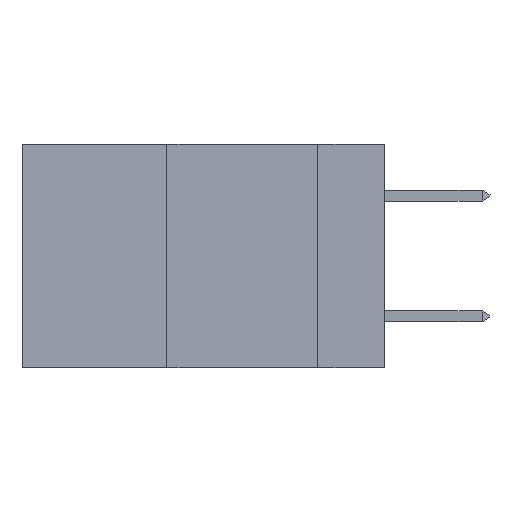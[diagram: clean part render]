
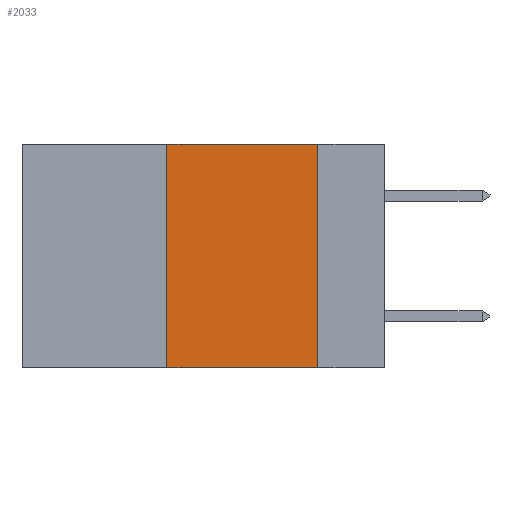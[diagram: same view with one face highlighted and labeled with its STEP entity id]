
A CAD part, left-side view. The second image highlights one B-rep face of the part: STEP entity #2033.
In plain terms, the highlighted planar face has unit normal (-1, 0, 0).
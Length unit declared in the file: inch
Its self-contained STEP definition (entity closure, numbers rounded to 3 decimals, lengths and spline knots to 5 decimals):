
#476 = VECTOR ( 'NONE', #6105, 39.37008 ) ;
#523 = CARTESIAN_POINT ( 'NONE',  ( 0., 0.11, 0. ) ) ;
#810 = ORIENTED_EDGE ( 'NONE', *, *, #3979, .F. ) ;
#1506 = DIRECTION ( 'NONE',  ( 0., 0., -1. ) ) ;
#2033 = ADVANCED_FACE ( 'NONE', ( #2945 ), #10459, .F. ) ;
#2602 = CARTESIAN_POINT ( 'NONE',  ( 0., 0.11, 0. ) ) ;
#2945 = FACE_OUTER_BOUND ( 'NONE', #3031, .T. ) ;
#3031 = EDGE_LOOP ( 'NONE', ( #9887, #810, #5860, #4939 ) ) ;
#3814 = DIRECTION ( 'NONE',  ( 0., -1., 0. ) ) ;
#3979 = EDGE_CURVE ( 'NONE', #7374, #7402, #9338, .T. ) ;
#4024 = VECTOR ( 'NONE', #5511, 39.37008 ) ;
#4125 = VECTOR ( 'NONE', #8876, 39.37008 ) ;
#4846 = EDGE_CURVE ( 'NONE', #8097, #7374, #6092, .T. ) ;
#4939 = ORIENTED_EDGE ( 'NONE', *, *, #6793, .T. ) ;
#5511 = DIRECTION ( 'NONE',  ( 0., 0., 1. ) ) ;
#5563 = CARTESIAN_POINT ( 'NONE',  ( 0., 0.6, 0. ) ) ;
#5622 = VERTEX_POINT ( 'NONE', #10888 ) ;
#5860 = ORIENTED_EDGE ( 'NONE', *, *, #4846, .F. ) ;
#6067 = CARTESIAN_POINT ( 'NONE',  ( 0., 0.36, -0.37 ) ) ;
#6092 = LINE ( 'NONE', #10984, #4024 ) ;
#6105 = DIRECTION ( 'NONE',  ( 0., 0., -1. ) ) ;
#6523 = CARTESIAN_POINT ( 'NONE',  ( 0., 0.6, -0.37 ) ) ;
#6793 = EDGE_CURVE ( 'NONE', #8097, #5622, #10842, .T. ) ;
#7257 = VECTOR ( 'NONE', #3814, 39.37008 ) ;
#7374 = VERTEX_POINT ( 'NONE', #7757 ) ;
#7402 = VERTEX_POINT ( 'NONE', #2602 ) ;
#7448 = LINE ( 'NONE', #523, #476 ) ;
#7757 = CARTESIAN_POINT ( 'NONE',  ( 0., 0.36, 0. ) ) ;
#8097 = VERTEX_POINT ( 'NONE', #6067 ) ;
#8160 = EDGE_CURVE ( 'NONE', #7402, #5622, #7448, .T. ) ;
#8876 = DIRECTION ( 'NONE',  ( 0., -1., 0. ) ) ;
#9103 = AXIS2_PLACEMENT_3D ( 'NONE', #10654, #10418, #1506 ) ;
#9338 = LINE ( 'NONE', #5563, #7257 ) ;
#9887 = ORIENTED_EDGE ( 'NONE', *, *, #8160, .F. ) ;
#10418 = DIRECTION ( 'NONE',  ( 1., 0., 0. ) ) ;
#10459 = PLANE ( 'NONE',  #9103 ) ;
#10654 = CARTESIAN_POINT ( 'NONE',  ( 0., 0.6, 0. ) ) ;
#10842 = LINE ( 'NONE', #6523, #4125 ) ;
#10888 = CARTESIAN_POINT ( 'NONE',  ( 0., 0.11, -0.37 ) ) ;
#10984 = CARTESIAN_POINT ( 'NONE',  ( 0., 0.36, 0. ) ) ;
